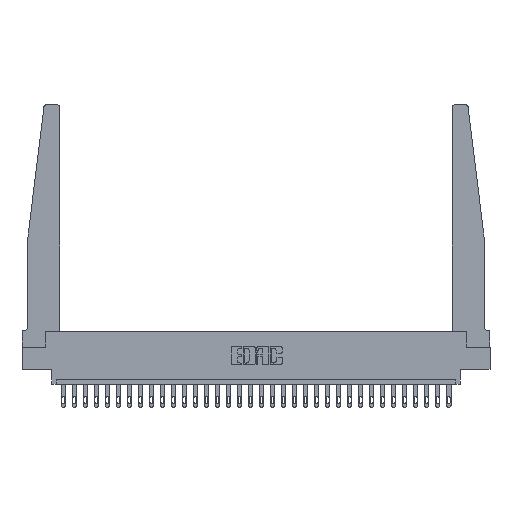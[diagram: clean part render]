
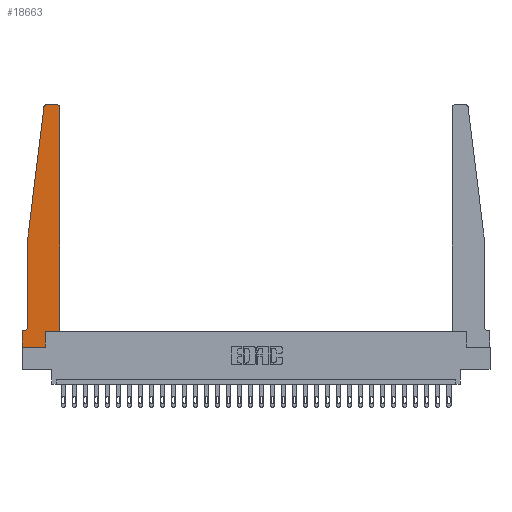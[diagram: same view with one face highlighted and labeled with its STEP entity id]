
A CAD part, top view. The second image highlights one B-rep face of the part: STEP entity #18663.
In plain terms, the highlighted planar face has unit normal (0, 0, 1).
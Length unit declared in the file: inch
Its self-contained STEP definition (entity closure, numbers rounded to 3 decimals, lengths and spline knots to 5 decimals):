
#236 = EDGE_LOOP ( 'NONE', ( #23918, #26346, #18106, #14816, #2939, #2481, #23197, #10317, #18120, #17065, #11069, #1434 ) ) ;
#531 = DIRECTION ( 'NONE',  ( 1., 0., 0. ) ) ;
#738 = VERTEX_POINT ( 'NONE', #2052 ) ;
#970 = VERTEX_POINT ( 'NONE', #10878 ) ;
#1100 = VERTEX_POINT ( 'NONE', #19626 ) ;
#1434 = ORIENTED_EDGE ( 'NONE', *, *, #19436, .T. ) ;
#2052 = CARTESIAN_POINT ( 'NONE',  ( 0., 0.1875, 0.37 ) ) ;
#2217 = DIRECTION ( 'NONE',  ( 1., 0., 0. ) ) ;
#2481 = ORIENTED_EDGE ( 'NONE', *, *, #23540, .T. ) ;
#2512 = VERTEX_POINT ( 'NONE', #23608 ) ;
#2572 = VECTOR ( 'NONE', #12902, 39.37008 ) ;
#2677 = CIRCLE ( 'NONE', #24726, 0.03 ) ;
#2939 = ORIENTED_EDGE ( 'NONE', *, *, #5649, .T. ) ;
#3130 = CARTESIAN_POINT ( 'NONE',  ( 0.24675, 2.72367, 0.37 ) ) ;
#4444 = PLANE ( 'NONE',  #23785 ) ;
#4962 = CARTESIAN_POINT ( 'NONE',  ( 0.27653, 2.72, 0.37 ) ) ;
#5144 = CARTESIAN_POINT ( 'NONE',  ( 0.065, 0.2375, 0.37 ) ) ;
#5410 = LINE ( 'NONE', #22554, #6812 ) ;
#5649 = EDGE_CURVE ( 'NONE', #27487, #16704, #7120, .T. ) ;
#5831 = EDGE_CURVE ( 'NONE', #7176, #27487, #23602, .T. ) ;
#6434 = VECTOR ( 'NONE', #17908, 39.37008 ) ;
#6462 = DIRECTION ( 'NONE',  ( 1., 0., 0. ) ) ;
#6601 = CARTESIAN_POINT ( 'NONE',  ( 0.065, 1.25, 0.37 ) ) ;
#6812 = VECTOR ( 'NONE', #18653, 39.37008 ) ;
#6915 = EDGE_CURVE ( 'NONE', #13065, #2512, #5410, .T. ) ;
#7120 = CIRCLE ( 'NONE', #23224, 0.05 ) ;
#7129 = LINE ( 'NONE', #9139, #6434 ) ;
#7176 = VERTEX_POINT ( 'NONE', #27252 ) ;
#7237 = CARTESIAN_POINT ( 'NONE',  ( 0.425, 2.72, 0.37 ) ) ;
#7364 = CARTESIAN_POINT ( 'NONE',  ( 0.395, 2.72, 0.37 ) ) ;
#9139 = CARTESIAN_POINT ( 'NONE',  ( 0.065, 0.1875, 0.37 ) ) ;
#9713 = EDGE_CURVE ( 'NONE', #970, #22320, #13649, .T. ) ;
#9902 = CARTESIAN_POINT ( 'NONE',  ( 0.425, 0.18, 0.37 ) ) ;
#9909 = EDGE_CURVE ( 'NONE', #22320, #15722, #12337, .T. ) ;
#10126 = EDGE_CURVE ( 'NONE', #2512, #23619, #23770, .T. ) ;
#10186 = DIRECTION ( 'NONE',  ( 0., 1., 0. ) ) ;
#10317 = ORIENTED_EDGE ( 'NONE', *, *, #18387, .T. ) ;
#10526 = VECTOR ( 'NONE', #18482, 39.37008 ) ;
#10878 = CARTESIAN_POINT ( 'NONE',  ( 0.2605, 0.18, 0.37 ) ) ;
#10897 = LINE ( 'NONE', #6601, #2572 ) ;
#11045 = DIRECTION ( 'NONE',  ( 0., 0., 1. ) ) ;
#11069 = ORIENTED_EDGE ( 'NONE', *, *, #9909, .T. ) ;
#12337 = LINE ( 'NONE', #23480, #14579 ) ;
#12902 = DIRECTION ( 'NONE',  ( -0.122, -0.992, 0. ) ) ;
#13065 = VERTEX_POINT ( 'NONE', #22307 ) ;
#13602 = AXIS2_PLACEMENT_3D ( 'NONE', #4962, #20209, #531 ) ;
#13649 = LINE ( 'NONE', #9902, #19713 ) ;
#14149 = VECTOR ( 'NONE', #23078, 39.37008 ) ;
#14330 = EDGE_CURVE ( 'NONE', #23619, #7176, #10897, .T. ) ;
#14579 = VECTOR ( 'NONE', #10186, 39.37008 ) ;
#14816 = ORIENTED_EDGE ( 'NONE', *, *, #5831, .T. ) ;
#15100 = CARTESIAN_POINT ( 'NONE',  ( 0., 0., 0.37 ) ) ;
#15312 = CARTESIAN_POINT ( 'NONE',  ( 0.015, 0.1875, 0.37 ) ) ;
#15722 = VERTEX_POINT ( 'NONE', #7237 ) ;
#15928 = DIRECTION ( 'NONE',  ( -1., 0., 0. ) ) ;
#16704 = VERTEX_POINT ( 'NONE', #15312 ) ;
#16786 = VECTOR ( 'NONE', #27639, 39.37008 ) ;
#17065 = ORIENTED_EDGE ( 'NONE', *, *, #9713, .T. ) ;
#17908 = DIRECTION ( 'NONE',  ( -1., 0., 0. ) ) ;
#18106 = ORIENTED_EDGE ( 'NONE', *, *, #14330, .T. ) ;
#18120 = ORIENTED_EDGE ( 'NONE', *, *, #27737, .T. ) ;
#18205 = CARTESIAN_POINT ( 'NONE',  ( 0.2605, 0.18, 0.37 ) ) ;
#18387 = EDGE_CURVE ( 'NONE', #26201, #1100, #21907, .T. ) ;
#18482 = DIRECTION ( 'NONE',  ( 0., 1., 0. ) ) ;
#18598 = LINE ( 'NONE', #18889, #14149 ) ;
#18653 = DIRECTION ( 'NONE',  ( -1., 0., 0. ) ) ;
#18663 = ADVANCED_FACE ( 'NONE', ( #25216 ), #4444, .T. ) ;
#18889 = CARTESIAN_POINT ( 'NONE',  ( 0., 0., 0.37 ) ) ;
#19436 = EDGE_CURVE ( 'NONE', #15722, #13065, #2677, .T. ) ;
#19626 = CARTESIAN_POINT ( 'NONE',  ( 0.2605, 0., 0.37 ) ) ;
#19713 = VECTOR ( 'NONE', #22760, 39.37008 ) ;
#20152 = DIRECTION ( 'NONE',  ( 0., 0., 1. ) ) ;
#20209 = DIRECTION ( 'NONE',  ( 0., 0., 1. ) ) ;
#20507 = LINE ( 'NONE', #18205, #10526 ) ;
#20591 = DIRECTION ( 'NONE',  ( 1., 0., 0. ) ) ;
#20990 = CARTESIAN_POINT ( 'NONE',  ( 0.015, 0.2375, 0.37 ) ) ;
#21426 = CARTESIAN_POINT ( 'NONE',  ( 0.065, 1.25, 0.37 ) ) ;
#21907 = LINE ( 'NONE', #15100, #27471 ) ;
#22307 = CARTESIAN_POINT ( 'NONE',  ( 0.395, 2.75, 0.37 ) ) ;
#22320 = VERTEX_POINT ( 'NONE', #25599 ) ;
#22554 = CARTESIAN_POINT ( 'NONE',  ( 0.25, 2.75, 0.37 ) ) ;
#22760 = DIRECTION ( 'NONE',  ( 1., 0., 0. ) ) ;
#23078 = DIRECTION ( 'NONE',  ( 0., -1., 0. ) ) ;
#23197 = ORIENTED_EDGE ( 'NONE', *, *, #26174, .T. ) ;
#23224 = AXIS2_PLACEMENT_3D ( 'NONE', #20990, #25040, #15928 ) ;
#23480 = CARTESIAN_POINT ( 'NONE',  ( 0.425, 0.18, 0.37 ) ) ;
#23540 = EDGE_CURVE ( 'NONE', #16704, #738, #7129, .T. ) ;
#23602 = LINE ( 'NONE', #21426, #16786 ) ;
#23608 = CARTESIAN_POINT ( 'NONE',  ( 0.27653, 2.75, 0.37 ) ) ;
#23619 = VERTEX_POINT ( 'NONE', #3130 ) ;
#23654 = CARTESIAN_POINT ( 'NONE',  ( 0., 0., 0.37 ) ) ;
#23770 = CIRCLE ( 'NONE', #13602, 0.03 ) ;
#23785 = AXIS2_PLACEMENT_3D ( 'NONE', #26495, #11045, #6462 ) ;
#23918 = ORIENTED_EDGE ( 'NONE', *, *, #6915, .T. ) ;
#24726 = AXIS2_PLACEMENT_3D ( 'NONE', #7364, #20152, #20591 ) ;
#25040 = DIRECTION ( 'NONE',  ( 0., 0., -1. ) ) ;
#25216 = FACE_OUTER_BOUND ( 'NONE', #236, .T. ) ;
#25599 = CARTESIAN_POINT ( 'NONE',  ( 0.425, 0.18, 0.37 ) ) ;
#26174 = EDGE_CURVE ( 'NONE', #738, #26201, #18598, .T. ) ;
#26201 = VERTEX_POINT ( 'NONE', #23654 ) ;
#26346 = ORIENTED_EDGE ( 'NONE', *, *, #10126, .T. ) ;
#26495 = CARTESIAN_POINT ( 'NONE',  ( 0., 0.1875, 0.37 ) ) ;
#27252 = CARTESIAN_POINT ( 'NONE',  ( 0.065, 1.25, 0.37 ) ) ;
#27471 = VECTOR ( 'NONE', #2217, 39.37008 ) ;
#27487 = VERTEX_POINT ( 'NONE', #5144 ) ;
#27639 = DIRECTION ( 'NONE',  ( 0., -1., 0. ) ) ;
#27737 = EDGE_CURVE ( 'NONE', #1100, #970, #20507, .T. ) ;
